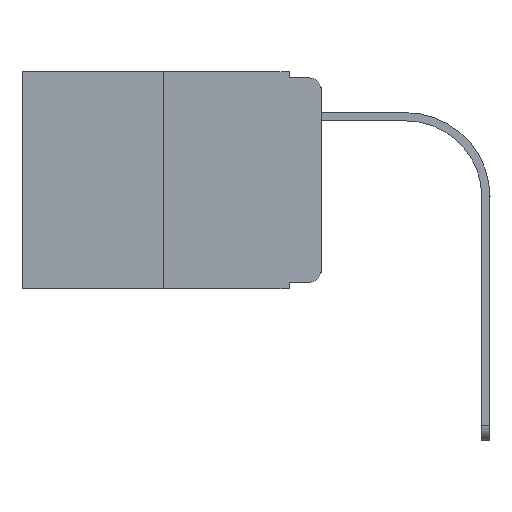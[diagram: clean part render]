
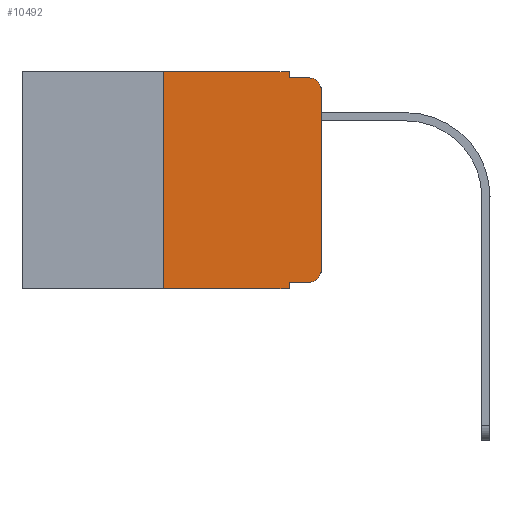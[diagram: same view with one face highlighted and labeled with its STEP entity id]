
A CAD part, left-side view. The second image highlights one B-rep face of the part: STEP entity #10492.
In plain terms, the highlighted planar face has unit normal (-1, 0, 0).
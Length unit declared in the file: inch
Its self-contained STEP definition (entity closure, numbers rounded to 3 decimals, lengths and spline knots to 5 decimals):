
#185 = CARTESIAN_POINT ( 'NONE',  ( 0., 0.051, 0. ) ) ;
#439 = DIRECTION ( 'NONE',  ( 0., 0., -1. ) ) ;
#926 = DIRECTION ( 'NONE',  ( 1., 0., 0. ) ) ;
#1150 = VECTOR ( 'NONE', #17632, 39.37008 ) ;
#1581 = LINE ( 'NONE', #17605, #11251 ) ;
#2560 = EDGE_CURVE ( 'NONE', #6670, #7265, #3805, .T. ) ;
#2576 = ORIENTED_EDGE ( 'NONE', *, *, #15118, .T. ) ;
#2854 = FACE_OUTER_BOUND ( 'NONE', #8856, .T. ) ;
#3285 = CARTESIAN_POINT ( 'NONE',  ( 0., 0.473, 0. ) ) ;
#3473 = EDGE_CURVE ( 'NONE', #9995, #17266, #13625, .T. ) ;
#3478 = CARTESIAN_POINT ( 'NONE',  ( 0., 0., -0.313 ) ) ;
#3795 = CARTESIAN_POINT ( 'NONE',  ( 0., 0.051, -0.333 ) ) ;
#3805 = LINE ( 'NONE', #10018, #1150 ) ;
#3986 = DIRECTION ( 'NONE',  ( 0., -1., 0. ) ) ;
#5058 = CIRCLE ( 'NONE', #13719, 0.02 ) ;
#5921 = LINE ( 'NONE', #25226, #9577 ) ;
#6161 = VERTEX_POINT ( 'NONE', #19708 ) ;
#6508 = DIRECTION ( 'NONE',  ( 0., 0., 1. ) ) ;
#6670 = VERTEX_POINT ( 'NONE', #3478 ) ;
#6788 = ORIENTED_EDGE ( 'NONE', *, *, #2560, .T. ) ;
#7146 = AXIS2_PLACEMENT_3D ( 'NONE', #16141, #19765, #11751 ) ;
#7265 = VERTEX_POINT ( 'NONE', #13727 ) ;
#8207 = VERTEX_POINT ( 'NONE', #17794 ) ;
#8736 = DIRECTION ( 'NONE',  ( 0., -1., 0. ) ) ;
#8856 = EDGE_LOOP ( 'NONE', ( #6788, #20833, #12648, #17995, #16905, #24356, #12038, #8943, #17407, #2576 ) ) ;
#8865 = CARTESIAN_POINT ( 'NONE',  ( 0., 0.25, 0. ) ) ;
#8943 = ORIENTED_EDGE ( 'NONE', *, *, #17541, .F. ) ;
#9577 = VECTOR ( 'NONE', #3986, 39.37008 ) ;
#9911 = CARTESIAN_POINT ( 'NONE',  ( 0., 0.02, -0.01 ) ) ;
#9995 = VERTEX_POINT ( 'NONE', #22428 ) ;
#10018 = CARTESIAN_POINT ( 'NONE',  ( 0., 0., 0. ) ) ;
#10056 = VERTEX_POINT ( 'NONE', #16978 ) ;
#10067 = LINE ( 'NONE', #17938, #17533 ) ;
#10492 = ADVANCED_FACE ( 'NONE', ( #2854 ), #22794, .F. ) ;
#11251 = VECTOR ( 'NONE', #25264, 39.37008 ) ;
#11751 = DIRECTION ( 'NONE',  ( 0., 0., -1. ) ) ;
#12038 = ORIENTED_EDGE ( 'NONE', *, *, #15308, .T. ) ;
#12507 = EDGE_CURVE ( 'NONE', #6161, #9995, #21123, .T. ) ;
#12648 = ORIENTED_EDGE ( 'NONE', *, *, #25302, .F. ) ;
#13196 = VECTOR ( 'NONE', #6508, 39.37008 ) ;
#13625 = LINE ( 'NONE', #185, #14673 ) ;
#13651 = VECTOR ( 'NONE', #15684, 39.37008 ) ;
#13719 = AXIS2_PLACEMENT_3D ( 'NONE', #16205, #16077, #23986 ) ;
#13727 = CARTESIAN_POINT ( 'NONE',  ( 0., 0., -0.03 ) ) ;
#14173 = VERTEX_POINT ( 'NONE', #24489 ) ;
#14249 = CARTESIAN_POINT ( 'NONE',  ( 0., 0.051, -0.333 ) ) ;
#14673 = VECTOR ( 'NONE', #439, 39.37008 ) ;
#15118 = EDGE_CURVE ( 'NONE', #8207, #6670, #5058, .T. ) ;
#15308 = EDGE_CURVE ( 'NONE', #10056, #14173, #1581, .T. ) ;
#15684 = DIRECTION ( 'NONE',  ( 0., -1., 0. ) ) ;
#15810 = LINE ( 'NONE', #14249, #13651 ) ;
#15826 = EDGE_CURVE ( 'NONE', #7265, #21852, #18296, .T. ) ;
#16077 = DIRECTION ( 'NONE',  ( -1., 0., 0. ) ) ;
#16141 = CARTESIAN_POINT ( 'NONE',  ( 0., 0.02, -0.03 ) ) ;
#16205 = CARTESIAN_POINT ( 'NONE',  ( 0., 0.02, -0.313 ) ) ;
#16905 = ORIENTED_EDGE ( 'NONE', *, *, #12507, .F. ) ;
#16978 = CARTESIAN_POINT ( 'NONE',  ( 0., 0.25, -0.343 ) ) ;
#17266 = VERTEX_POINT ( 'NONE', #20925 ) ;
#17407 = ORIENTED_EDGE ( 'NONE', *, *, #22299, .T. ) ;
#17533 = VECTOR ( 'NONE', #20129, 39.37008 ) ;
#17541 = EDGE_CURVE ( 'NONE', #23057, #14173, #10067, .T. ) ;
#17605 = CARTESIAN_POINT ( 'NONE',  ( 0., 0.473, -0.343 ) ) ;
#17632 = DIRECTION ( 'NONE',  ( 0., 0., 1. ) ) ;
#17794 = CARTESIAN_POINT ( 'NONE',  ( 0., 0.02, -0.333 ) ) ;
#17938 = CARTESIAN_POINT ( 'NONE',  ( 0., 0.051, 0. ) ) ;
#17995 = ORIENTED_EDGE ( 'NONE', *, *, #3473, .F. ) ;
#18296 = CIRCLE ( 'NONE', #7146, 0.02 ) ;
#18635 = CARTESIAN_POINT ( 'NONE',  ( 0., 0.473, 0. ) ) ;
#19315 = AXIS2_PLACEMENT_3D ( 'NONE', #18635, #926, #22664 ) ;
#19708 = CARTESIAN_POINT ( 'NONE',  ( 0., 0.25, 0. ) ) ;
#19765 = DIRECTION ( 'NONE',  ( -1., 0., 0. ) ) ;
#19785 = VECTOR ( 'NONE', #8736, 39.37008 ) ;
#20129 = DIRECTION ( 'NONE',  ( 0., 0., -1. ) ) ;
#20833 = ORIENTED_EDGE ( 'NONE', *, *, #15826, .T. ) ;
#20925 = CARTESIAN_POINT ( 'NONE',  ( 0., 0.051, -0.01 ) ) ;
#21123 = LINE ( 'NONE', #3285, #19785 ) ;
#21852 = VERTEX_POINT ( 'NONE', #9911 ) ;
#22088 = EDGE_CURVE ( 'NONE', #10056, #6161, #24762, .T. ) ;
#22299 = EDGE_CURVE ( 'NONE', #23057, #8207, #15810, .T. ) ;
#22428 = CARTESIAN_POINT ( 'NONE',  ( 0., 0.051, 0. ) ) ;
#22664 = DIRECTION ( 'NONE',  ( 0., 0., -1. ) ) ;
#22794 = PLANE ( 'NONE',  #19315 ) ;
#23057 = VERTEX_POINT ( 'NONE', #3795 ) ;
#23986 = DIRECTION ( 'NONE',  ( 0., 0., -1. ) ) ;
#24356 = ORIENTED_EDGE ( 'NONE', *, *, #22088, .F. ) ;
#24489 = CARTESIAN_POINT ( 'NONE',  ( 0., 0.051, -0.343 ) ) ;
#24762 = LINE ( 'NONE', #8865, #13196 ) ;
#25226 = CARTESIAN_POINT ( 'NONE',  ( 0., 0.051, -0.01 ) ) ;
#25264 = DIRECTION ( 'NONE',  ( 0., -1., 0. ) ) ;
#25302 = EDGE_CURVE ( 'NONE', #17266, #21852, #5921, .T. ) ;
